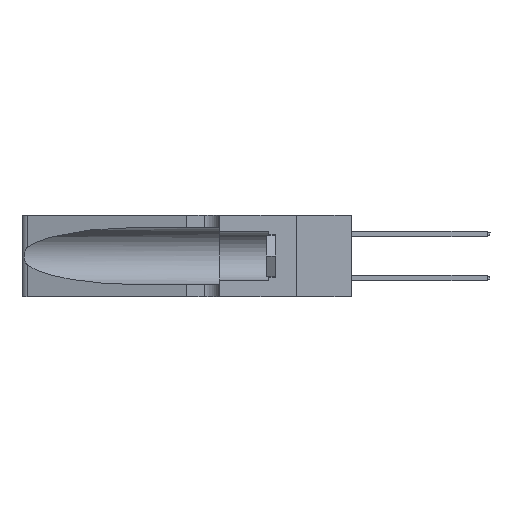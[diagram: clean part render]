
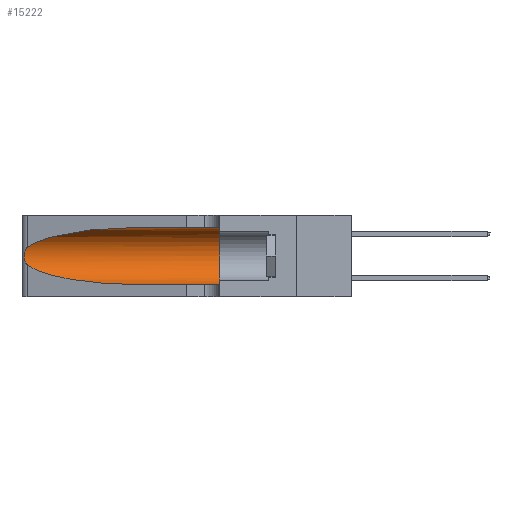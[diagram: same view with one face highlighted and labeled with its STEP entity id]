
A CAD part, left-side view. The second image highlights one B-rep face of the part: STEP entity #15222.
In plain terms, the highlighted cylindrical face has radius 3.308 mm (diameter 6.617 mm), a partial arc.
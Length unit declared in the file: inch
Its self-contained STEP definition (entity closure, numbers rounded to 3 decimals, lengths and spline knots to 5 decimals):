
#247 = EDGE_CURVE ( 'NONE', #3109, #13294, #10308, .T. ) ;
#905 = AXIS2_PLACEMENT_3D ( 'NONE', #1093, #16623, #14941 ) ;
#908 = CARTESIAN_POINT ( 'NONE',  ( 0.26018, 1.23835, 0.19895 ) ) ;
#1093 = CARTESIAN_POINT ( 'NONE',  ( 0.1305, 1.61858, 0.185 ) ) ;
#1173 = CARTESIAN_POINT ( 'NONE',  ( 0.1305, 1.61858, 0.31525 ) ) ;
#1381 = CARTESIAN_POINT ( 'NONE',  ( 0.25487, 1.22718, 0.22369 ) ) ;
#1739 = CARTESIAN_POINT ( 'NONE',  ( 0.1305, 0.72297, 0.05475 ) ) ;
#1906 =( BOUNDED_CURVE ( )  B_SPLINE_CURVE ( 3, ( #10359, #20455, #12123, #1739 ),
 .UNSPECIFIED., .F., .F. ) 
 B_SPLINE_CURVE_WITH_KNOTS ( ( 4, 4 ),
 ( 3.44316, 4.71239 ),
 .UNSPECIFIED. ) 
 CURVE ( )  GEOMETRIC_REPRESENTATION_ITEM ( )  RATIONAL_B_SPLINE_CURVE ( ( 1., 0.87, 0.87, 1. ) ) 
 REPRESENTATION_ITEM ( '' )  );
#2495 = ORIENTED_EDGE ( 'NONE', *, *, #9836, .T. ) ;
#2588 = LINE ( 'NONE', #21793, #15788 ) ;
#2704 = CARTESIAN_POINT ( 'NONE',  ( 0.26075, 1.23896, 0.178 ) ) ;
#3109 = VERTEX_POINT ( 'NONE', #18204 ) ;
#3253 = DIRECTION ( 'NONE',  ( 0., -1., 0. ) ) ;
#3420 = VERTEX_POINT ( 'NONE', #19057 ) ;
#4421 = CARTESIAN_POINT ( 'NONE',  ( 0.25856, 1.23593, 0.16098 ) ) ;
#4885 = DIRECTION ( 'NONE',  ( 0., 1., 0. ) ) ;
#5930 =( BOUNDED_CURVE ( )  B_SPLINE_CURVE ( 3, ( #6528, #21809, #11769, #1381 ),
 .UNSPECIFIED., .F., .F. ) 
 B_SPLINE_CURVE_WITH_KNOTS ( ( 4, 4 ),
 ( 1.5708, 2.84003 ),
 .UNSPECIFIED. ) 
 CURVE ( )  GEOMETRIC_REPRESENTATION_ITEM ( )  RATIONAL_B_SPLINE_CURVE ( ( 1., 0.87, 0.87, 1. ) ) 
 REPRESENTATION_ITEM ( '' )  );
#6099 = CARTESIAN_POINT ( 'NONE',  ( 0.25487, 1.22718, 0.22369 ) ) ;
#6176 = CARTESIAN_POINT ( 'NONE',  ( 0.25639, 1.23186, 0.15144 ) ) ;
#6528 = CARTESIAN_POINT ( 'NONE',  ( 0.1305, 0.72297, 0.31525 ) ) ;
#7329 = ORIENTED_EDGE ( 'NONE', *, *, #16714, .T. ) ;
#7410 = EDGE_LOOP ( 'NONE', ( #2495, #19260, #14922, #7329, #10366, #12898 ) ) ;
#7891 = CARTESIAN_POINT ( 'NONE',  ( 0.25487, 1.22718, 0.14631 ) ) ;
#9503 = CARTESIAN_POINT ( 'NONE',  ( 0.25555, 1.22994, 0.2215 ) ) ;
#9583 = CARTESIAN_POINT ( 'NONE',  ( 0.25639, 1.23184, 0.21858 ) ) ;
#9689 = EDGE_CURVE ( 'NONE', #3420, #11157, #9951, .T. ) ;
#9836 = EDGE_CURVE ( 'NONE', #3109, #3420, #5930, .T. ) ;
#9951 = B_SPLINE_CURVE_WITH_KNOTS ( 'NONE', 3,
 ( #6099, #9503, #9583, #21384, #11332, #908, #13082, #2704, #14782, #4421, #16450, #6176, #18115, #7891 ),
 .UNSPECIFIED., .F., .F.,
 ( 4, 2, 2, 2, 2, 2, 4 ),
 ( 0., 0.00027, 0.00053, 0.00107, 0.0016, 0.00187, 0.00214 ),
 .UNSPECIFIED. ) ;
#10003 = DIRECTION ( 'NONE',  ( 0., -1., 0. ) ) ;
#10308 = LINE ( 'NONE', #1173, #14886 ) ;
#10359 = CARTESIAN_POINT ( 'NONE',  ( 0.25487, 1.22718, 0.14631 ) ) ;
#10366 = ORIENTED_EDGE ( 'NONE', *, *, #21620, .F. ) ;
#11157 = VERTEX_POINT ( 'NONE', #17525 ) ;
#11332 = CARTESIAN_POINT ( 'NONE',  ( 0.25854, 1.2359, 0.20912 ) ) ;
#11605 = CIRCLE ( 'NONE', #17305, 0.13025 ) ;
#11769 = CARTESIAN_POINT ( 'NONE',  ( 0.2373, 1.15595, 0.28018 ) ) ;
#11821 = VERTEX_POINT ( 'NONE', #12212 ) ;
#12123 = CARTESIAN_POINT ( 'NONE',  ( 0.18966, 0.96281, 0.05475 ) ) ;
#12212 = CARTESIAN_POINT ( 'NONE',  ( 0.1305, 0.72297, 0.05475 ) ) ;
#12282 = EDGE_CURVE ( 'NONE', #11157, #11821, #1906, .T. ) ;
#12392 = CYLINDRICAL_SURFACE ( 'NONE', #905, 0.13025 ) ;
#12898 = ORIENTED_EDGE ( 'NONE', *, *, #247, .F. ) ;
#13082 = CARTESIAN_POINT ( 'NONE',  ( 0.26075, 1.23896, 0.19203 ) ) ;
#13294 = VERTEX_POINT ( 'NONE', #16367 ) ;
#14782 = CARTESIAN_POINT ( 'NONE',  ( 0.26017, 1.23833, 0.17102 ) ) ;
#14886 = VECTOR ( 'NONE', #3253, 39.37008 ) ;
#14922 = ORIENTED_EDGE ( 'NONE', *, *, #12282, .T. ) ;
#14939 = VERTEX_POINT ( 'NONE', #16040 ) ;
#14941 = DIRECTION ( 'NONE',  ( 0., 0., -1. ) ) ;
#15213 = CARTESIAN_POINT ( 'NONE',  ( 0.1305, 0.35, 0.185 ) ) ;
#15222 = ADVANCED_FACE ( 'NONE', ( #21282 ), #12392, .F. ) ;
#15788 = VECTOR ( 'NONE', #10003, 39.37008 ) ;
#16040 = CARTESIAN_POINT ( 'NONE',  ( 0.1305, 0.35, 0.05475 ) ) ;
#16367 = CARTESIAN_POINT ( 'NONE',  ( 0.1305, 0.35, 0.31525 ) ) ;
#16450 = CARTESIAN_POINT ( 'NONE',  ( 0.25789, 1.23486, 0.15765 ) ) ;
#16623 = DIRECTION ( 'NONE',  ( 0., -1., 0. ) ) ;
#16714 = EDGE_CURVE ( 'NONE', #11821, #14939, #2588, .T. ) ;
#16889 = DIRECTION ( 'NONE',  ( 0., 0., 1. ) ) ;
#17305 = AXIS2_PLACEMENT_3D ( 'NONE', #15213, #4885, #16889 ) ;
#17525 = CARTESIAN_POINT ( 'NONE',  ( 0.25487, 1.22718, 0.14631 ) ) ;
#18115 = CARTESIAN_POINT ( 'NONE',  ( 0.25555, 1.22993, 0.14849 ) ) ;
#18204 = CARTESIAN_POINT ( 'NONE',  ( 0.1305, 0.72297, 0.31525 ) ) ;
#19057 = CARTESIAN_POINT ( 'NONE',  ( 0.25487, 1.22718, 0.22369 ) ) ;
#19260 = ORIENTED_EDGE ( 'NONE', *, *, #9689, .T. ) ;
#20455 = CARTESIAN_POINT ( 'NONE',  ( 0.2373, 1.15595, 0.08982 ) ) ;
#21282 = FACE_OUTER_BOUND ( 'NONE', #7410, .T. ) ;
#21384 = CARTESIAN_POINT ( 'NONE',  ( 0.25787, 1.23484, 0.2124 ) ) ;
#21620 = EDGE_CURVE ( 'NONE', #13294, #14939, #11605, .T. ) ;
#21793 = CARTESIAN_POINT ( 'NONE',  ( 0.1305, 1.61858, 0.05475 ) ) ;
#21809 = CARTESIAN_POINT ( 'NONE',  ( 0.18966, 0.96281, 0.31525 ) ) ;
